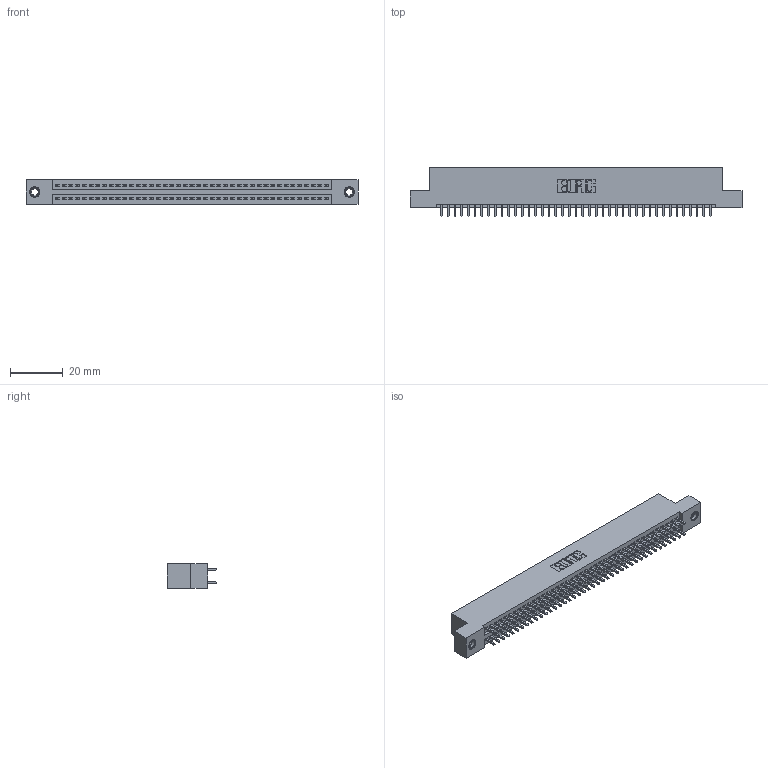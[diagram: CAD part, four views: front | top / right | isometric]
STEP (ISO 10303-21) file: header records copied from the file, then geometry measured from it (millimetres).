
FILE_DESCRIPTION (( 'STEP AP203' ), '1' );
FILE_NAME ('395-082-521-207.STEP', '2018-11-28T06:48:14', ( '' ), ( '' ), 'SwSTEP 2.0', 'SolidWorks 2016', '' );
FILE_SCHEMA (( 'CONFIG_CONTROL_DESIGN' ));
Length unit declared in the file: inch
Products named in the file (4): 345 Part_Flush Mounting Lugs - 0.156 Dia-TI; 345-292-001_345-293-121; 345-250-001_345-250-005-103; 395-082-521-207
Assembly tree (85 placements, depth 2):
  395-082-521-207
    345 Part_Flush Mounting Lugs - 0.156 Dia-TI
    345-292-001_345-293-121  x82
    345-250-001_345-250-005-103  x2
Bounding box: 125.35 x 18.72 x 9.4 mm (x, y, z)
Volume: 12120.3 mm3; surface area: 17706.5 mm2
Topology: 85 solids, 85 shells, 4286 faces, 12695 edges, 8346 vertices
Faces by surface type: plane 2818, cylinder 1452, cone 12, torus 4
Entity records: 33508 total; most frequent: CARTESIAN_POINT 5599, ORIENTED_EDGE 5526, DIRECTION 4965, EDGE_CURVE 2763, LINE 2447, VECTOR 2447, VERTEX_POINT 1836, AXIS2_PLACEMENT_3D 1259
